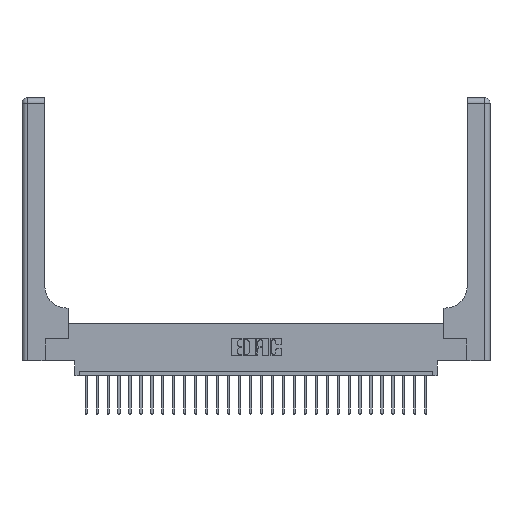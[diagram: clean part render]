
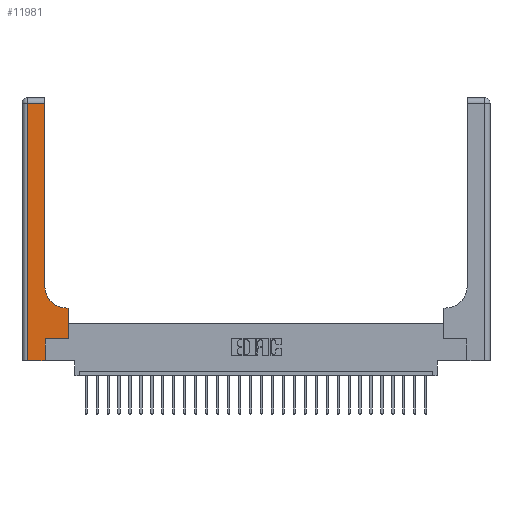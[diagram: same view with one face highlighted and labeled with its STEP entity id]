
A CAD part, top view. The second image highlights one B-rep face of the part: STEP entity #11981.
In plain terms, the highlighted planar face has unit normal (0, 0, 1).
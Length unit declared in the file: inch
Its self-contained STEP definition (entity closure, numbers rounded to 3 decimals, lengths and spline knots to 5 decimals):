
#5 = CARTESIAN_POINT ( 'NONE',  ( 0.265, 0., 0.37 ) ) ;
#117 = EDGE_CURVE ( 'NONE', #8513, #16585, #342, .T. ) ;
#342 = LINE ( 'NONE', #8672, #26576 ) ;
#471 = VECTOR ( 'NONE', #3055, 39.37008 ) ;
#1339 = CARTESIAN_POINT ( 'NONE',  ( 0.26, 0.85, 0.37 ) ) ;
#2015 = ORIENTED_EDGE ( 'NONE', *, *, #13038, .T. ) ;
#2512 = LINE ( 'NONE', #10836, #3564 ) ;
#2881 = VERTEX_POINT ( 'NONE', #5 ) ;
#3055 = DIRECTION ( 'NONE',  ( -1., 0., 0. ) ) ;
#3095 = LINE ( 'NONE', #21007, #12731 ) ;
#3564 = VECTOR ( 'NONE', #11371, 39.37008 ) ;
#4352 = DIRECTION ( 'NONE',  ( 1., 0., 0. ) ) ;
#4534 = CARTESIAN_POINT ( 'NONE',  ( 0.528, 0.6, 0.37 ) ) ;
#4642 = CARTESIAN_POINT ( 'NONE',  ( 0., 3., 0.37 ) ) ;
#4798 = ORIENTED_EDGE ( 'NONE', *, *, #15059, .T. ) ;
#5828 = ORIENTED_EDGE ( 'NONE', *, *, #14116, .T. ) ;
#6390 = LINE ( 'NONE', #18515, #21211 ) ;
#6431 = VERTEX_POINT ( 'NONE', #19687 ) ;
#6810 = VERTEX_POINT ( 'NONE', #15959 ) ;
#6845 = DIRECTION ( 'NONE',  ( 0., 0., -1. ) ) ;
#7024 = ORIENTED_EDGE ( 'NONE', *, *, #117, .T. ) ;
#7044 = AXIS2_PLACEMENT_3D ( 'NONE', #4642, #6845, #15135 ) ;
#8513 = VERTEX_POINT ( 'NONE', #1339 ) ;
#8672 = CARTESIAN_POINT ( 'NONE',  ( 0.26, 3., 0.37 ) ) ;
#9754 = CARTESIAN_POINT ( 'NONE',  ( 0.26, 2.94, 0.37 ) ) ;
#10579 = CIRCLE ( 'NONE', #25813, 0.25 ) ;
#10674 = ORIENTED_EDGE ( 'NONE', *, *, #12823, .T. ) ;
#10836 = CARTESIAN_POINT ( 'NONE',  ( 0.265, 0.25, 0.37 ) ) ;
#11161 = ORIENTED_EDGE ( 'NONE', *, *, #11197, .T. ) ;
#11197 = EDGE_CURVE ( 'NONE', #16585, #20226, #15588, .T. ) ;
#11371 = DIRECTION ( 'NONE',  ( 1., 0., 0. ) ) ;
#11561 = VERTEX_POINT ( 'NONE', #4534 ) ;
#11981 = ADVANCED_FACE ( 'NONE', ( #21141 ), #25362, .F. ) ;
#12102 = EDGE_LOOP ( 'NONE', ( #7024, #11161, #5828, #10674, #26935, #4798, #23273, #2015, #13245 ) ) ;
#12424 = LINE ( 'NONE', #12561, #17486 ) ;
#12561 = CARTESIAN_POINT ( 'NONE',  ( 0.06, 3., 0.37 ) ) ;
#12731 = VECTOR ( 'NONE', #15758, 39.37008 ) ;
#12823 = EDGE_CURVE ( 'NONE', #14572, #2881, #16887, .T. ) ;
#13038 = EDGE_CURVE ( 'NONE', #11561, #6810, #3095, .T. ) ;
#13168 = VECTOR ( 'NONE', #4352, 39.37008 ) ;
#13245 = ORIENTED_EDGE ( 'NONE', *, *, #15625, .T. ) ;
#13813 = CARTESIAN_POINT ( 'NONE',  ( 0., 2.94, 0.37 ) ) ;
#14116 = EDGE_CURVE ( 'NONE', #20226, #14572, #12424, .T. ) ;
#14572 = VERTEX_POINT ( 'NONE', #18256 ) ;
#15059 = EDGE_CURVE ( 'NONE', #19994, #6431, #2512, .T. ) ;
#15135 = DIRECTION ( 'NONE',  ( -1., 0., 0. ) ) ;
#15588 = LINE ( 'NONE', #13813, #471 ) ;
#15625 = EDGE_CURVE ( 'NONE', #6810, #8513, #10579, .T. ) ;
#15758 = DIRECTION ( 'NONE',  ( -1., 0., 0. ) ) ;
#15959 = CARTESIAN_POINT ( 'NONE',  ( 0.51, 0.6, 0.37 ) ) ;
#16585 = VERTEX_POINT ( 'NONE', #9754 ) ;
#16887 = LINE ( 'NONE', #18396, #13168 ) ;
#16969 = DIRECTION ( 'NONE',  ( 0., 1., 0. ) ) ;
#17486 = VECTOR ( 'NONE', #22653, 39.37008 ) ;
#17582 = CARTESIAN_POINT ( 'NONE',  ( 0.51, 0.85, 0.37 ) ) ;
#18256 = CARTESIAN_POINT ( 'NONE',  ( 0.06, 0., 0.37 ) ) ;
#18396 = CARTESIAN_POINT ( 'NONE',  ( 0., 0., 0.37 ) ) ;
#18515 = CARTESIAN_POINT ( 'NONE',  ( 0.528, 0.25, 0.37 ) ) ;
#19175 = CARTESIAN_POINT ( 'NONE',  ( 0.265, 0., 0.37 ) ) ;
#19687 = CARTESIAN_POINT ( 'NONE',  ( 0.528, 0.25, 0.37 ) ) ;
#19994 = VERTEX_POINT ( 'NONE', #25663 ) ;
#20226 = VERTEX_POINT ( 'NONE', #21956 ) ;
#20771 = VECTOR ( 'NONE', #25169, 39.37008 ) ;
#21007 = CARTESIAN_POINT ( 'NONE',  ( 0.26, 0.6, 0.37 ) ) ;
#21141 = FACE_OUTER_BOUND ( 'NONE', #12102, .T. ) ;
#21211 = VECTOR ( 'NONE', #24785, 39.37008 ) ;
#21220 = LINE ( 'NONE', #19175, #20771 ) ;
#21956 = CARTESIAN_POINT ( 'NONE',  ( 0.06, 2.94, 0.37 ) ) ;
#22653 = DIRECTION ( 'NONE',  ( 0., -1., 0. ) ) ;
#23273 = ORIENTED_EDGE ( 'NONE', *, *, #25460, .T. ) ;
#24785 = DIRECTION ( 'NONE',  ( 0., 1., 0. ) ) ;
#25169 = DIRECTION ( 'NONE',  ( 0., 1., 0. ) ) ;
#25362 = PLANE ( 'NONE',  #7044 ) ;
#25460 = EDGE_CURVE ( 'NONE', #6431, #11561, #6390, .T. ) ;
#25518 = DIRECTION ( 'NONE',  ( 0., 0., -1. ) ) ;
#25663 = CARTESIAN_POINT ( 'NONE',  ( 0.265, 0.25, 0.37 ) ) ;
#25813 = AXIS2_PLACEMENT_3D ( 'NONE', #17582, #25518, #25918 ) ;
#25870 = EDGE_CURVE ( 'NONE', #2881, #19994, #21220, .T. ) ;
#25918 = DIRECTION ( 'NONE',  ( 1., 0., 0. ) ) ;
#26576 = VECTOR ( 'NONE', #16969, 39.37008 ) ;
#26935 = ORIENTED_EDGE ( 'NONE', *, *, #25870, .T. ) ;
